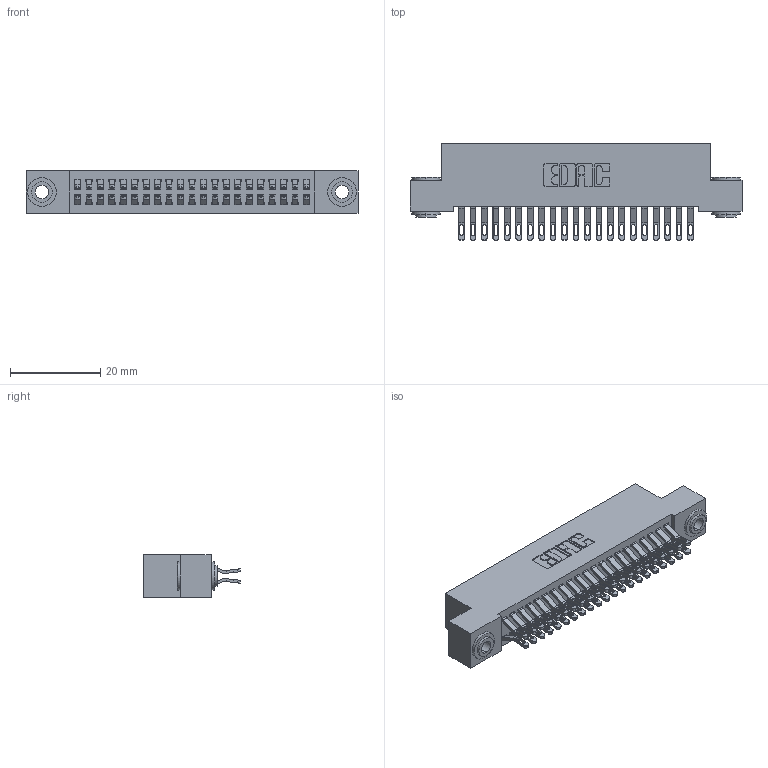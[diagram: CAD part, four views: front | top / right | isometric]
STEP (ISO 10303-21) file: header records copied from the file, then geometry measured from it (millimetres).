
FILE_DESCRIPTION (( 'STEP AP203' ), '1' );
FILE_NAME ('342-042-555-203.STEP', '2019-10-02T18:10:11', ( '' ), ( '' ), 'SwSTEP 2.0', 'SolidWorks 2016', '' );
FILE_SCHEMA (( 'CONFIG_CONTROL_DESIGN' ));
Length unit declared in the file: inch
Products named in the file (4): 342 Part_.156 TH; 345-292-001_555 Tail; 342-250-002_345-250-002-102; 342-042-555-203
Assembly tree (45 placements, depth 2):
  342-042-555-203
    342 Part_.156 TH
    345-292-001_555 Tail  x42
    342-250-002_345-250-002-102  x2
Bounding box: 73.66 x 21.47 x 9.4 mm (x, y, z)
Volume: 6658.5 mm3; surface area: 10941.3 mm2
Topology: 45 solids, 45 shells, 2584 faces, 8061 edges, 5370 vertices
Faces by surface type: plane 1504, cylinder 1072, cone 8
Entity records: 17070 total; most frequent: CARTESIAN_POINT 2863, ORIENTED_EDGE 2762, DIRECTION 2487, EDGE_CURVE 1381, VECTOR 1209, LINE 1209, VERTEX_POINT 918, AXIS2_PLACEMENT_3D 639
